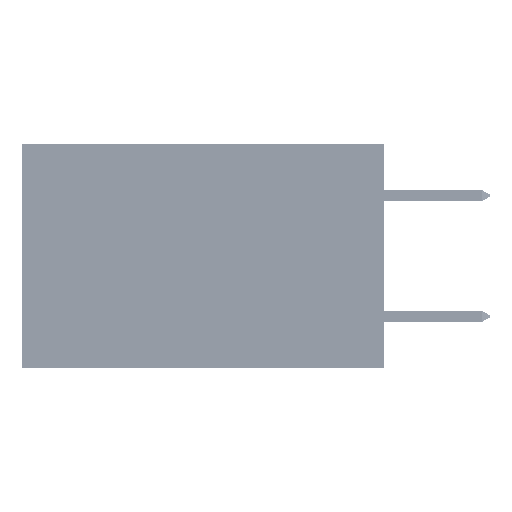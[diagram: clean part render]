
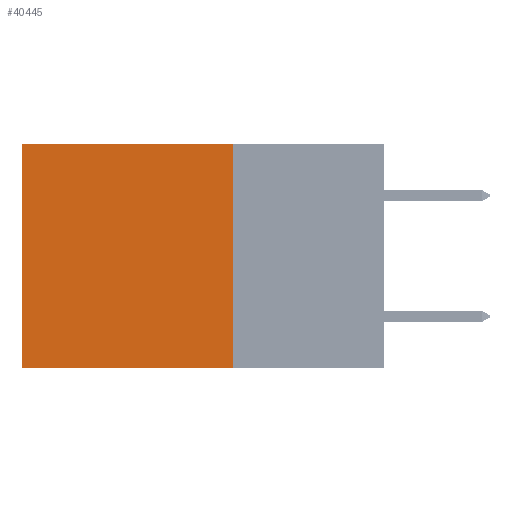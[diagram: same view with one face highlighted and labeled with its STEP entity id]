
A CAD part, left-side view. The second image highlights one B-rep face of the part: STEP entity #40445.
In plain terms, the highlighted planar face has unit normal (-1, 0, 0).
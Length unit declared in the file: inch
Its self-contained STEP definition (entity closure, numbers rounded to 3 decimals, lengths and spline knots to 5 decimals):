
#1625 = LINE ( 'NONE', #2594, #42194 ) ;
#2037 = FACE_OUTER_BOUND ( 'NONE', #17831, .T. ) ;
#2314 = VECTOR ( 'NONE', #22640, 39.37008 ) ;
#2594 = CARTESIAN_POINT ( 'NONE',  ( 0.2875, 0.25, -0.37 ) ) ;
#2982 = VERTEX_POINT ( 'NONE', #33897 ) ;
#4918 = DIRECTION ( 'NONE',  ( 0., 0., -1. ) ) ;
#4955 = DIRECTION ( 'NONE',  ( 1., 0., 0. ) ) ;
#5631 = CARTESIAN_POINT ( 'NONE',  ( 0.2875, 0.25, 0. ) ) ;
#6003 = LINE ( 'NONE', #21274, #35496 ) ;
#8508 = VERTEX_POINT ( 'NONE', #26771 ) ;
#13200 = PLANE ( 'NONE',  #36996 ) ;
#13961 = ORIENTED_EDGE ( 'NONE', *, *, #42993, .T. ) ;
#15071 = EDGE_CURVE ( 'NONE', #8508, #23200, #38817, .T. ) ;
#15881 = DIRECTION ( 'NONE',  ( 0., 0., -1. ) ) ;
#17117 = VECTOR ( 'NONE', #4918, 39.37008 ) ;
#17831 = EDGE_LOOP ( 'NONE', ( #45814, #19778, #28388, #13961 ) ) ;
#18670 = CARTESIAN_POINT ( 'NONE',  ( 0.2875, 0.25, -0.37 ) ) ;
#19493 = CARTESIAN_POINT ( 'NONE',  ( 0.2875, 0.6, 0. ) ) ;
#19778 = ORIENTED_EDGE ( 'NONE', *, *, #36970, .F. ) ;
#21274 = CARTESIAN_POINT ( 'NONE',  ( 0.2875, 0.25, 0. ) ) ;
#22640 = DIRECTION ( 'NONE',  ( 0., 0., -1. ) ) ;
#22866 = EDGE_CURVE ( 'NONE', #2982, #47142, #40549, .T. ) ;
#23200 = VERTEX_POINT ( 'NONE', #18670 ) ;
#26730 = CARTESIAN_POINT ( 'NONE',  ( 0.2875, 0.6, -0.37 ) ) ;
#26771 = CARTESIAN_POINT ( 'NONE',  ( 0.2875, 0.25, 0. ) ) ;
#26992 = CARTESIAN_POINT ( 'NONE',  ( 0.2875, 0.25, 0. ) ) ;
#28388 = ORIENTED_EDGE ( 'NONE', *, *, #15071, .F. ) ;
#32139 = DIRECTION ( 'NONE',  ( 0., 1., 0. ) ) ;
#33897 = CARTESIAN_POINT ( 'NONE',  ( 0.2875, 0.6, 0. ) ) ;
#35496 = VECTOR ( 'NONE', #39180, 39.37008 ) ;
#36970 = EDGE_CURVE ( 'NONE', #23200, #47142, #1625, .T. ) ;
#36996 = AXIS2_PLACEMENT_3D ( 'NONE', #26992, #4955, #15881 ) ;
#38817 = LINE ( 'NONE', #5631, #17117 ) ;
#39180 = DIRECTION ( 'NONE',  ( 0., 1., 0. ) ) ;
#40445 = ADVANCED_FACE ( 'NONE', ( #2037 ), #13200, .F. ) ;
#40549 = LINE ( 'NONE', #19493, #2314 ) ;
#42194 = VECTOR ( 'NONE', #32139, 39.37008 ) ;
#42993 = EDGE_CURVE ( 'NONE', #8508, #2982, #6003, .T. ) ;
#45814 = ORIENTED_EDGE ( 'NONE', *, *, #22866, .T. ) ;
#47142 = VERTEX_POINT ( 'NONE', #26730 ) ;
